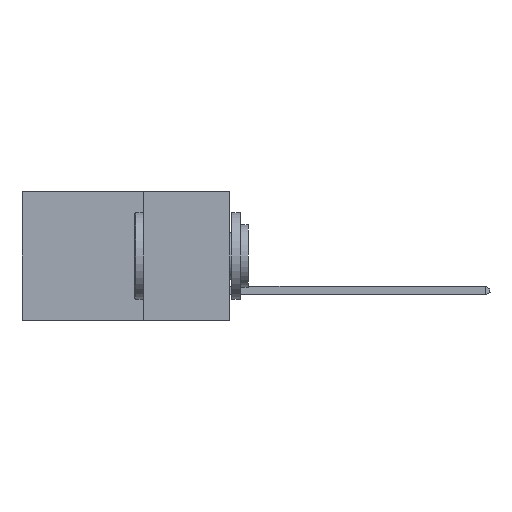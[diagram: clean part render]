
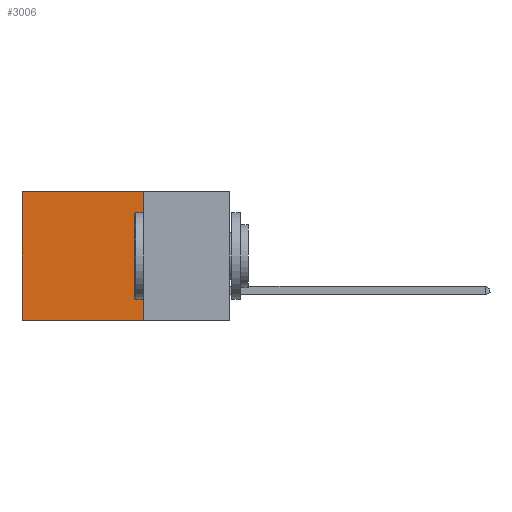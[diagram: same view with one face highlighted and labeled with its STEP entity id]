
A CAD part, left-side view. The second image highlights one B-rep face of the part: STEP entity #3006.
In plain terms, the highlighted planar face has unit normal (-1, 0, 0).
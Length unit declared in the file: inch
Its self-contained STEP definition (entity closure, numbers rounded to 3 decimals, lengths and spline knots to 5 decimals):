
#904 = CARTESIAN_POINT ( 'NONE',  ( 0.298, 0.25, 0. ) ) ;
#1403 = ORIENTED_EDGE ( 'NONE', *, *, #4198, .F. ) ;
#2007 = CARTESIAN_POINT ( 'NONE',  ( 0.298, 0.6, 0. ) ) ;
#2403 = LINE ( 'NONE', #904, #5874 ) ;
#2767 = PLANE ( 'NONE',  #5702 ) ;
#2867 = CARTESIAN_POINT ( 'NONE',  ( 0.298, 0.25, 0. ) ) ;
#3006 = ADVANCED_FACE ( 'NONE', ( #14310 ), #2767, .F. ) ;
#3203 = VERTEX_POINT ( 'NONE', #12938 ) ;
#3596 = CARTESIAN_POINT ( 'NONE',  ( 0.298, 0.6, 0. ) ) ;
#3736 = DIRECTION ( 'NONE',  ( 0., 0., -1. ) ) ;
#4198 = EDGE_CURVE ( 'NONE', #11312, #3203, #11146, .T. ) ;
#4221 = CARTESIAN_POINT ( 'NONE',  ( 0.298, 0.25, -0.37 ) ) ;
#5224 = VECTOR ( 'NONE', #3736, 39.37008 ) ;
#5232 = VERTEX_POINT ( 'NONE', #14086 ) ;
#5702 = AXIS2_PLACEMENT_3D ( 'NONE', #2867, #12843, #7145 ) ;
#5800 = CARTESIAN_POINT ( 'NONE',  ( 0.298, 0.25, 0. ) ) ;
#5870 = ORIENTED_EDGE ( 'NONE', *, *, #10364, .T. ) ;
#5874 = VECTOR ( 'NONE', #8707, 39.37008 ) ;
#6118 = EDGE_CURVE ( 'NONE', #5232, #11312, #2403, .T. ) ;
#7145 = DIRECTION ( 'NONE',  ( 0., 0., -1. ) ) ;
#8707 = DIRECTION ( 'NONE',  ( 0., 0., -1. ) ) ;
#9266 = EDGE_CURVE ( 'NONE', #5232, #9520, #10848, .T. ) ;
#9520 = VERTEX_POINT ( 'NONE', #2007 ) ;
#9916 = ORIENTED_EDGE ( 'NONE', *, *, #9266, .T. ) ;
#10251 = DIRECTION ( 'NONE',  ( 0., 1., 0. ) ) ;
#10364 = EDGE_CURVE ( 'NONE', #9520, #3203, #11168, .T. ) ;
#10443 = VECTOR ( 'NONE', #13160, 39.37008 ) ;
#10848 = LINE ( 'NONE', #5800, #13811 ) ;
#11146 = LINE ( 'NONE', #13260, #10443 ) ;
#11168 = LINE ( 'NONE', #3596, #5224 ) ;
#11312 = VERTEX_POINT ( 'NONE', #4221 ) ;
#11955 = EDGE_LOOP ( 'NONE', ( #5870, #1403, #13727, #9916 ) ) ;
#12843 = DIRECTION ( 'NONE',  ( 1., 0., 0. ) ) ;
#12938 = CARTESIAN_POINT ( 'NONE',  ( 0.298, 0.6, -0.37 ) ) ;
#13160 = DIRECTION ( 'NONE',  ( 0., 1., 0. ) ) ;
#13260 = CARTESIAN_POINT ( 'NONE',  ( 0.298, 0.25, -0.37 ) ) ;
#13727 = ORIENTED_EDGE ( 'NONE', *, *, #6118, .F. ) ;
#13811 = VECTOR ( 'NONE', #10251, 39.37008 ) ;
#14086 = CARTESIAN_POINT ( 'NONE',  ( 0.298, 0.25, 0. ) ) ;
#14310 = FACE_OUTER_BOUND ( 'NONE', #11955, .T. ) ;
